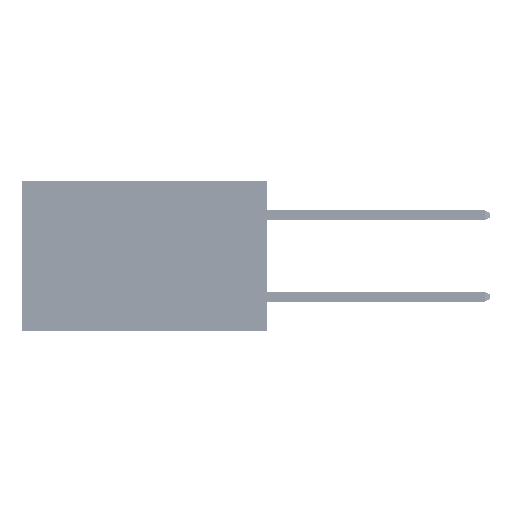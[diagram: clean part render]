
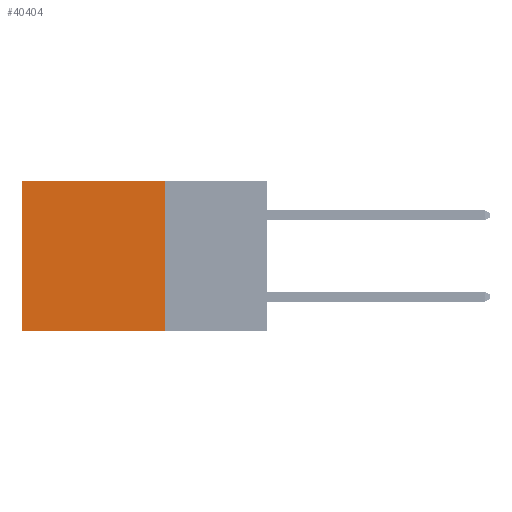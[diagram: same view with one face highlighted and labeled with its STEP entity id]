
A CAD part, left-side view. The second image highlights one B-rep face of the part: STEP entity #40404.
In plain terms, the highlighted planar face has unit normal (-1, 0, 0).
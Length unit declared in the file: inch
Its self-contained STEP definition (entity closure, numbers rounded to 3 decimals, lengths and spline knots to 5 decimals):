
#3456 = EDGE_LOOP ( 'NONE', ( #38296, #20822, #24649, #13709 ) ) ;
#5203 = EDGE_CURVE ( 'NONE', #11884, #13991, #14149, .T. ) ;
#5783 = DIRECTION ( 'NONE',  ( 0., 1., 0. ) ) ;
#6312 = CARTESIAN_POINT ( 'NONE',  ( 0.2875, 0.25, 0. ) ) ;
#10129 = DIRECTION ( 'NONE',  ( 0., 0., -1. ) ) ;
#11035 = CARTESIAN_POINT ( 'NONE',  ( 0.2875, 0.6, 0. ) ) ;
#11884 = VERTEX_POINT ( 'NONE', #28352 ) ;
#11913 = CARTESIAN_POINT ( 'NONE',  ( 0.2875, 0.6, -0.37 ) ) ;
#13709 = ORIENTED_EDGE ( 'NONE', *, *, #17875, .T. ) ;
#13991 = VERTEX_POINT ( 'NONE', #44822 ) ;
#14149 = LINE ( 'NONE', #29736, #31394 ) ;
#16069 = LINE ( 'NONE', #31408, #23302 ) ;
#17123 = LINE ( 'NONE', #27694, #35648 ) ;
#17875 = EDGE_CURVE ( 'NONE', #11884, #42212, #17123, .T. ) ;
#20822 = ORIENTED_EDGE ( 'NONE', *, *, #29175, .F. ) ;
#20983 = VECTOR ( 'NONE', #5783, 39.37008 ) ;
#23302 = VECTOR ( 'NONE', #38707, 39.37008 ) ;
#24649 = ORIENTED_EDGE ( 'NONE', *, *, #5203, .F. ) ;
#24681 = DIRECTION ( 'NONE',  ( 0., 1., 0. ) ) ;
#24936 = LINE ( 'NONE', #40258, #20983 ) ;
#27694 = CARTESIAN_POINT ( 'NONE',  ( 0.2875, 0.25, 0. ) ) ;
#28352 = CARTESIAN_POINT ( 'NONE',  ( 0.2875, 0.25, 0. ) ) ;
#29175 = EDGE_CURVE ( 'NONE', #13991, #46340, #24936, .T. ) ;
#29229 = DIRECTION ( 'NONE',  ( 0., 0., -1. ) ) ;
#29736 = CARTESIAN_POINT ( 'NONE',  ( 0.2875, 0.25, 0. ) ) ;
#30383 = PLANE ( 'NONE',  #43792 ) ;
#31394 = VECTOR ( 'NONE', #10129, 39.37008 ) ;
#31408 = CARTESIAN_POINT ( 'NONE',  ( 0.2875, 0.6, 0. ) ) ;
#34155 = DIRECTION ( 'NONE',  ( 1., 0., 0. ) ) ;
#35648 = VECTOR ( 'NONE', #24681, 39.37008 ) ;
#38296 = ORIENTED_EDGE ( 'NONE', *, *, #47414, .T. ) ;
#38707 = DIRECTION ( 'NONE',  ( 0., 0., -1. ) ) ;
#40258 = CARTESIAN_POINT ( 'NONE',  ( 0.2875, 0.25, -0.37 ) ) ;
#40404 = ADVANCED_FACE ( 'NONE', ( #48343 ), #30383, .F. ) ;
#42212 = VERTEX_POINT ( 'NONE', #11035 ) ;
#43792 = AXIS2_PLACEMENT_3D ( 'NONE', #6312, #34155, #29229 ) ;
#44822 = CARTESIAN_POINT ( 'NONE',  ( 0.2875, 0.25, -0.37 ) ) ;
#46340 = VERTEX_POINT ( 'NONE', #11913 ) ;
#47414 = EDGE_CURVE ( 'NONE', #42212, #46340, #16069, .T. ) ;
#48343 = FACE_OUTER_BOUND ( 'NONE', #3456, .T. ) ;
